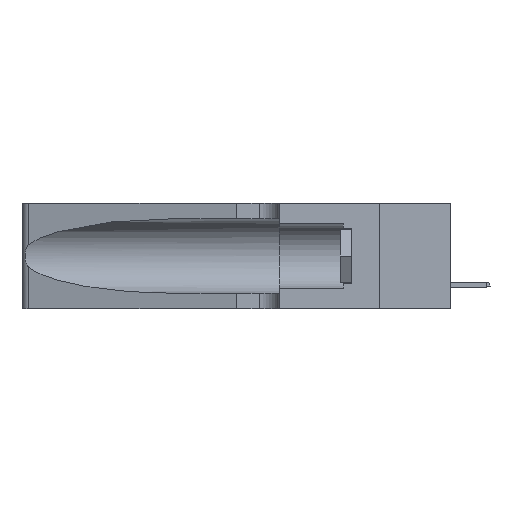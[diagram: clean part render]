
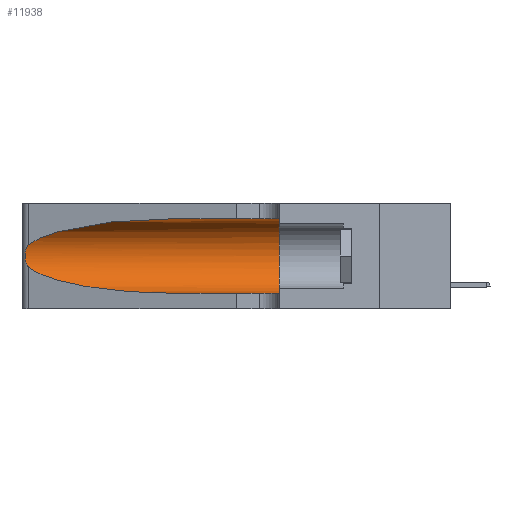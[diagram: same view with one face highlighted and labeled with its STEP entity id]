
A CAD part, left-side view. The second image highlights one B-rep face of the part: STEP entity #11938.
In plain terms, the highlighted cylindrical face has radius 3.308 mm (diameter 6.617 mm), a partial arc.
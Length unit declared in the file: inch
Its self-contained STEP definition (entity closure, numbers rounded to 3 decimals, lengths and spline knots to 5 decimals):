
#19 = DIRECTION ( 'NONE',  ( 0., -1., 0. ) ) ;
#1071 = CARTESIAN_POINT ( 'NONE',  ( 0.1305, 0.72297, 0.31525 ) ) ;
#1403 = CARTESIAN_POINT ( 'NONE',  ( 0.25787, 1.23484, 0.2124 ) ) ;
#1421 =( BOUNDED_CURVE ( )  B_SPLINE_CURVE ( 3, ( #18439, #2934, #7483, #1490 ),
 .UNSPECIFIED., .F., .T. ) 
 B_SPLINE_CURVE_WITH_KNOTS ( ( 4, 4 ),
 ( 3.44316, 4.71239 ),
 .UNSPECIFIED. ) 
 CURVE ( )  GEOMETRIC_REPRESENTATION_ITEM ( )  RATIONAL_B_SPLINE_CURVE ( ( 1., 0.87, 0.87, 1. ) ) 
 REPRESENTATION_ITEM ( '' )  );
#1465 = DIRECTION ( 'NONE',  ( 0., 1., 0. ) ) ;
#1490 = CARTESIAN_POINT ( 'NONE',  ( 0.1305, 0.72297, 0.05475 ) ) ;
#1503 = CARTESIAN_POINT ( 'NONE',  ( 0.26018, 1.23835, 0.19895 ) ) ;
#1506 = EDGE_CURVE ( 'NONE', #10069, #16428, #14218, .T. ) ;
#1541 = B_SPLINE_CURVE_WITH_KNOTS ( 'NONE', 3,
 ( #12512, #15678, #6346, #1403, #9222, #1503, #12203, #18453, #4569, #1605, #10862, #9122, #13842, #12307 ),
 .UNSPECIFIED., .F., .F.,
 ( 4, 2, 2, 2, 2, 2, 4 ),
 ( 0., 0.00027, 0.00053, 0.00107, 0.0016, 0.00187, 0.00214 ),
 .UNSPECIFIED. ) ;
#1605 = CARTESIAN_POINT ( 'NONE',  ( 0.25856, 1.23593, 0.16098 ) ) ;
#1733 = CARTESIAN_POINT ( 'NONE',  ( 0.1305, 0.35, 0.05475 ) ) ;
#1998 = CARTESIAN_POINT ( 'NONE',  ( 0.1305, 1.61858, 0.31525 ) ) ;
#2049 = EDGE_CURVE ( 'NONE', #7684, #4686, #18428, .T. ) ;
#2739 = CARTESIAN_POINT ( 'NONE',  ( 0.1305, 0.72297, 0.31525 ) ) ;
#2934 = CARTESIAN_POINT ( 'NONE',  ( 0.2373, 1.15595, 0.08982 ) ) ;
#3408 = EDGE_CURVE ( 'NONE', #16428, #4686, #8677, .T. ) ;
#4569 = CARTESIAN_POINT ( 'NONE',  ( 0.26017, 1.23833, 0.17102 ) ) ;
#4664 = ORIENTED_EDGE ( 'NONE', *, *, #12199, .T. ) ;
#4686 = VERTEX_POINT ( 'NONE', #1733 ) ;
#4810 = CYLINDRICAL_SURFACE ( 'NONE', #8423, 0.13025 ) ;
#4913 = EDGE_CURVE ( 'NONE', #10069, #5164, #5610, .T. ) ;
#5008 = VECTOR ( 'NONE', #15549, 39.37008 ) ;
#5164 = VERTEX_POINT ( 'NONE', #17383 ) ;
#5610 =( BOUNDED_CURVE ( )  B_SPLINE_CURVE ( 3, ( #2739, #16636, #7388, #14968 ),
 .UNSPECIFIED., .F., .F. ) 
 B_SPLINE_CURVE_WITH_KNOTS ( ( 4, 4 ),
 ( 1.5708, 2.84003 ),
 .UNSPECIFIED. ) 
 CURVE ( )  GEOMETRIC_REPRESENTATION_ITEM ( )  RATIONAL_B_SPLINE_CURVE ( ( 1., 0.87, 0.87, 1. ) ) 
 REPRESENTATION_ITEM ( '' )  );
#6346 = CARTESIAN_POINT ( 'NONE',  ( 0.25639, 1.23184, 0.21858 ) ) ;
#6657 = ORIENTED_EDGE ( 'NONE', *, *, #3408, .F. ) ;
#6797 = CARTESIAN_POINT ( 'NONE',  ( 0.25487, 1.22718, 0.14631 ) ) ;
#7335 = VECTOR ( 'NONE', #17615, 39.37008 ) ;
#7388 = CARTESIAN_POINT ( 'NONE',  ( 0.2373, 1.15595, 0.28018 ) ) ;
#7483 = CARTESIAN_POINT ( 'NONE',  ( 0.18966, 0.96281, 0.05475 ) ) ;
#7684 = VERTEX_POINT ( 'NONE', #9787 ) ;
#8423 = AXIS2_PLACEMENT_3D ( 'NONE', #9358, #19, #15918 ) ;
#8677 = CIRCLE ( 'NONE', #9676, 0.13025 ) ;
#9122 = CARTESIAN_POINT ( 'NONE',  ( 0.25639, 1.23186, 0.15144 ) ) ;
#9191 = CARTESIAN_POINT ( 'NONE',  ( 0.1305, 1.61858, 0.05475 ) ) ;
#9222 = CARTESIAN_POINT ( 'NONE',  ( 0.25854, 1.2359, 0.20912 ) ) ;
#9236 = ORIENTED_EDGE ( 'NONE', *, *, #1506, .F. ) ;
#9358 = CARTESIAN_POINT ( 'NONE',  ( 0.1305, 1.61858, 0.185 ) ) ;
#9676 = AXIS2_PLACEMENT_3D ( 'NONE', #15542, #1465, #17300 ) ;
#9787 = CARTESIAN_POINT ( 'NONE',  ( 0.1305, 0.72297, 0.05475 ) ) ;
#10069 = VERTEX_POINT ( 'NONE', #1071 ) ;
#10205 = VERTEX_POINT ( 'NONE', #6797 ) ;
#10862 = CARTESIAN_POINT ( 'NONE',  ( 0.25789, 1.23486, 0.15765 ) ) ;
#11779 = CARTESIAN_POINT ( 'NONE',  ( 0.1305, 0.35, 0.31525 ) ) ;
#11938 = ADVANCED_FACE ( 'NONE', ( #17174 ), #4810, .F. ) ;
#12199 = EDGE_CURVE ( 'NONE', #10205, #7684, #1421, .T. ) ;
#12203 = CARTESIAN_POINT ( 'NONE',  ( 0.26075, 1.23896, 0.19203 ) ) ;
#12307 = CARTESIAN_POINT ( 'NONE',  ( 0.25487, 1.22718, 0.14631 ) ) ;
#12512 = CARTESIAN_POINT ( 'NONE',  ( 0.25487, 1.22718, 0.22369 ) ) ;
#13842 = CARTESIAN_POINT ( 'NONE',  ( 0.25555, 1.22993, 0.14849 ) ) ;
#14218 = LINE ( 'NONE', #1998, #7335 ) ;
#14968 = CARTESIAN_POINT ( 'NONE',  ( 0.25487, 1.22718, 0.22369 ) ) ;
#15542 = CARTESIAN_POINT ( 'NONE',  ( 0.1305, 0.35, 0.185 ) ) ;
#15549 = DIRECTION ( 'NONE',  ( 0., -1., 0. ) ) ;
#15678 = CARTESIAN_POINT ( 'NONE',  ( 0.25555, 1.22994, 0.2215 ) ) ;
#15918 = DIRECTION ( 'NONE',  ( 0., 0., -1. ) ) ;
#16257 = EDGE_CURVE ( 'NONE', #5164, #10205, #1541, .T. ) ;
#16428 = VERTEX_POINT ( 'NONE', #11779 ) ;
#16636 = CARTESIAN_POINT ( 'NONE',  ( 0.18966, 0.96281, 0.31525 ) ) ;
#16842 = ORIENTED_EDGE ( 'NONE', *, *, #16257, .T. ) ;
#17174 = FACE_OUTER_BOUND ( 'NONE', #17571, .T. ) ;
#17300 = DIRECTION ( 'NONE',  ( 0., 0., 1. ) ) ;
#17383 = CARTESIAN_POINT ( 'NONE',  ( 0.25487, 1.22718, 0.22369 ) ) ;
#17557 = ORIENTED_EDGE ( 'NONE', *, *, #4913, .T. ) ;
#17571 = EDGE_LOOP ( 'NONE', ( #17557, #16842, #4664, #19259, #6657, #9236 ) ) ;
#17615 = DIRECTION ( 'NONE',  ( 0., -1., 0. ) ) ;
#18428 = LINE ( 'NONE', #9191, #5008 ) ;
#18439 = CARTESIAN_POINT ( 'NONE',  ( 0.25487, 1.22718, 0.14631 ) ) ;
#18453 = CARTESIAN_POINT ( 'NONE',  ( 0.26075, 1.23896, 0.178 ) ) ;
#19259 = ORIENTED_EDGE ( 'NONE', *, *, #2049, .T. ) ;
